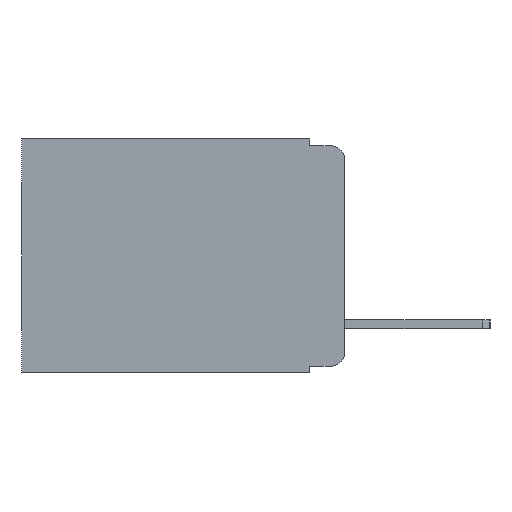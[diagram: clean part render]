
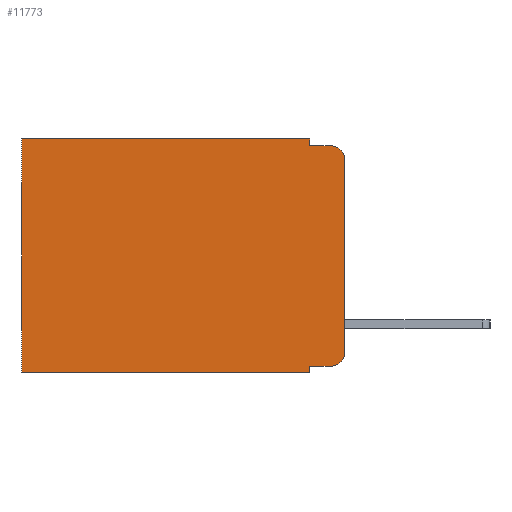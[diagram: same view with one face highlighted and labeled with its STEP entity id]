
A CAD part, left-side view. The second image highlights one B-rep face of the part: STEP entity #11773.
In plain terms, the highlighted planar face has unit normal (-1, 0, 0).
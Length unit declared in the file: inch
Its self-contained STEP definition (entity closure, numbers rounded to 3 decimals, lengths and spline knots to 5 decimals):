
#146 = CARTESIAN_POINT ( 'NONE',  ( 0.298, 0., 0. ) ) ;
#268 = DIRECTION ( 'NONE',  ( 0., 1., 0. ) ) ;
#336 = EDGE_CURVE ( 'NONE', #21962, #3129, #21704, .T. ) ;
#347 = ORIENTED_EDGE ( 'NONE', *, *, #4623, .F. ) ;
#1889 = DIRECTION ( 'NONE',  ( 0., 0., -1. ) ) ;
#1985 = ORIENTED_EDGE ( 'NONE', *, *, #21627, .T. ) ;
#2031 = LINE ( 'NONE', #2675, #11171 ) ;
#2633 = CARTESIAN_POINT ( 'NONE',  ( 0.298, 0.473, 0. ) ) ;
#2675 = CARTESIAN_POINT ( 'NONE',  ( 0.298, 0.051, -0.333 ) ) ;
#2895 = AXIS2_PLACEMENT_3D ( 'NONE', #18636, #8128, #20388 ) ;
#3129 = VERTEX_POINT ( 'NONE', #18533 ) ;
#3384 = CARTESIAN_POINT ( 'NONE',  ( 0.298, 0., -0.343 ) ) ;
#4450 = VERTEX_POINT ( 'NONE', #16372 ) ;
#4623 = EDGE_CURVE ( 'NONE', #5297, #4450, #12985, .T. ) ;
#4900 = LINE ( 'NONE', #6230, #18499 ) ;
#5243 = DIRECTION ( 'NONE',  ( 0., 1., 0. ) ) ;
#5272 = ORIENTED_EDGE ( 'NONE', *, *, #11919, .F. ) ;
#5297 = VERTEX_POINT ( 'NONE', #14542 ) ;
#5999 = AXIS2_PLACEMENT_3D ( 'NONE', #16396, #21590, #11235 ) ;
#6031 = VERTEX_POINT ( 'NONE', #8979 ) ;
#6183 = CARTESIAN_POINT ( 'NONE',  ( 0.298, 0.051, 0. ) ) ;
#6230 = CARTESIAN_POINT ( 'NONE',  ( 0.298, 0.051, 0. ) ) ;
#6807 = CIRCLE ( 'NONE', #8999, 0.02 ) ;
#7190 = ORIENTED_EDGE ( 'NONE', *, *, #8296, .T. ) ;
#7327 = VERTEX_POINT ( 'NONE', #20315 ) ;
#7643 = EDGE_LOOP ( 'NONE', ( #7848, #15636, #17365, #347, #17420, #1985, #9850, #5272, #20742, #7190 ) ) ;
#7848 = ORIENTED_EDGE ( 'NONE', *, *, #336, .F. ) ;
#8128 = DIRECTION ( 'NONE',  ( -1., 0., 0. ) ) ;
#8279 = LINE ( 'NONE', #13136, #21654 ) ;
#8296 = EDGE_CURVE ( 'NONE', #11363, #3129, #6807, .T. ) ;
#8882 = VECTOR ( 'NONE', #20884, 39.37008 ) ;
#8979 = CARTESIAN_POINT ( 'NONE',  ( 0.298, 0.02, -0.01 ) ) ;
#8999 = AXIS2_PLACEMENT_3D ( 'NONE', #9957, #22065, #11747 ) ;
#9429 = PLANE ( 'NONE',  #5999 ) ;
#9850 = ORIENTED_EDGE ( 'NONE', *, *, #15226, .F. ) ;
#9914 = DIRECTION ( 'NONE',  ( 0., 0., -1. ) ) ;
#9957 = CARTESIAN_POINT ( 'NONE',  ( 0.298, 0.02, -0.313 ) ) ;
#10084 = VERTEX_POINT ( 'NONE', #2633 ) ;
#10102 = CARTESIAN_POINT ( 'NONE',  ( 0.298, 0.02, -0.333 ) ) ;
#10385 = CARTESIAN_POINT ( 'NONE',  ( 0.298, 0.473, 0. ) ) ;
#10716 = EDGE_CURVE ( 'NONE', #21962, #6031, #16986, .T. ) ;
#11171 = VECTOR ( 'NONE', #17025, 39.37008 ) ;
#11235 = DIRECTION ( 'NONE',  ( 0., 0., -1. ) ) ;
#11363 = VERTEX_POINT ( 'NONE', #10102 ) ;
#11734 = VECTOR ( 'NONE', #12363, 39.37008 ) ;
#11747 = DIRECTION ( 'NONE',  ( 0., 0., -1. ) ) ;
#11773 = ADVANCED_FACE ( 'NONE', ( #13163 ), #9429, .F. ) ;
#11919 = EDGE_CURVE ( 'NONE', #13216, #7327, #4900, .T. ) ;
#12270 = LINE ( 'NONE', #19155, #11734 ) ;
#12363 = DIRECTION ( 'NONE',  ( 0., -1., 0. ) ) ;
#12985 = LINE ( 'NONE', #6183, #22603 ) ;
#13136 = CARTESIAN_POINT ( 'NONE',  ( 0.298, 0., 0. ) ) ;
#13163 = FACE_OUTER_BOUND ( 'NONE', #7643, .T. ) ;
#13216 = VERTEX_POINT ( 'NONE', #17045 ) ;
#14080 = VECTOR ( 'NONE', #5243, 39.37008 ) ;
#14542 = CARTESIAN_POINT ( 'NONE',  ( 0.298, 0.051, 0. ) ) ;
#15226 = EDGE_CURVE ( 'NONE', #7327, #19324, #22617, .T. ) ;
#15636 = ORIENTED_EDGE ( 'NONE', *, *, #10716, .T. ) ;
#16372 = CARTESIAN_POINT ( 'NONE',  ( 0.298, 0.051, -0.01 ) ) ;
#16396 = CARTESIAN_POINT ( 'NONE',  ( 0.298, 0., 0. ) ) ;
#16986 = CIRCLE ( 'NONE', #2895, 0.02 ) ;
#17025 = DIRECTION ( 'NONE',  ( 0., -1., 0. ) ) ;
#17045 = CARTESIAN_POINT ( 'NONE',  ( 0.298, 0.051, -0.333 ) ) ;
#17365 = ORIENTED_EDGE ( 'NONE', *, *, #22177, .F. ) ;
#17394 = VECTOR ( 'NONE', #19032, 39.37008 ) ;
#17420 = ORIENTED_EDGE ( 'NONE', *, *, #21836, .T. ) ;
#17765 = EDGE_CURVE ( 'NONE', #13216, #11363, #2031, .T. ) ;
#17921 = LINE ( 'NONE', #10385, #17394 ) ;
#18499 = VECTOR ( 'NONE', #9914, 39.37008 ) ;
#18533 = CARTESIAN_POINT ( 'NONE',  ( 0.298, 0., -0.313 ) ) ;
#18636 = CARTESIAN_POINT ( 'NONE',  ( 0.298, 0.02, -0.03 ) ) ;
#19032 = DIRECTION ( 'NONE',  ( 0., 0., -1. ) ) ;
#19155 = CARTESIAN_POINT ( 'NONE',  ( 0.298, 0.051, -0.01 ) ) ;
#19324 = VERTEX_POINT ( 'NONE', #20679 ) ;
#20315 = CARTESIAN_POINT ( 'NONE',  ( 0.298, 0.051, -0.343 ) ) ;
#20388 = DIRECTION ( 'NONE',  ( 0., 0., -1. ) ) ;
#20679 = CARTESIAN_POINT ( 'NONE',  ( 0.298, 0.473, -0.343 ) ) ;
#20742 = ORIENTED_EDGE ( 'NONE', *, *, #17765, .T. ) ;
#20884 = DIRECTION ( 'NONE',  ( 0., 0., -1. ) ) ;
#21590 = DIRECTION ( 'NONE',  ( 1., 0., 0. ) ) ;
#21627 = EDGE_CURVE ( 'NONE', #10084, #19324, #17921, .T. ) ;
#21654 = VECTOR ( 'NONE', #268, 39.37008 ) ;
#21704 = LINE ( 'NONE', #146, #8882 ) ;
#21836 = EDGE_CURVE ( 'NONE', #5297, #10084, #8279, .T. ) ;
#21962 = VERTEX_POINT ( 'NONE', #22028 ) ;
#22028 = CARTESIAN_POINT ( 'NONE',  ( 0.298, 0., -0.03 ) ) ;
#22065 = DIRECTION ( 'NONE',  ( -1., 0., 0. ) ) ;
#22177 = EDGE_CURVE ( 'NONE', #4450, #6031, #12270, .T. ) ;
#22603 = VECTOR ( 'NONE', #1889, 39.37008 ) ;
#22617 = LINE ( 'NONE', #3384, #14080 ) ;
